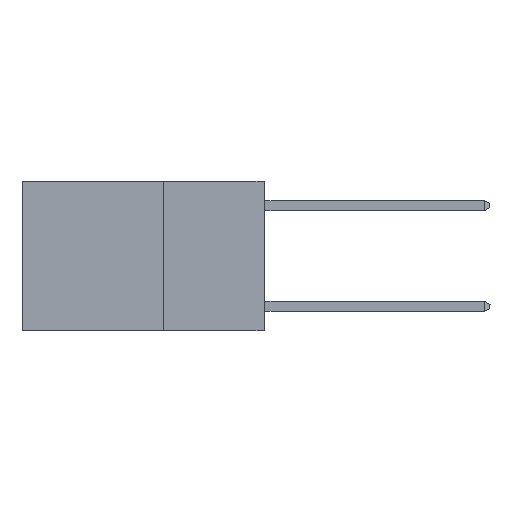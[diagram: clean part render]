
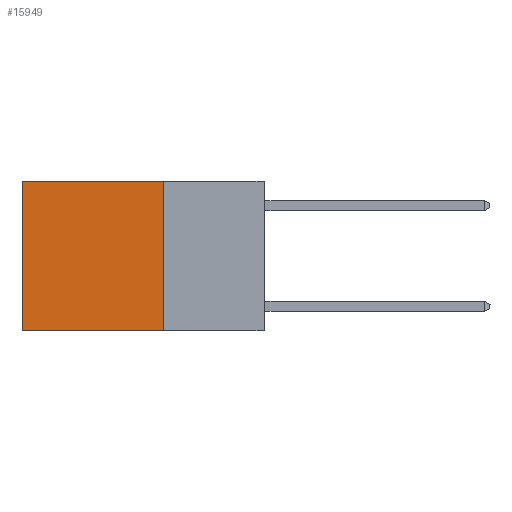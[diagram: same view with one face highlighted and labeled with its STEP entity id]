
A CAD part, left-side view. The second image highlights one B-rep face of the part: STEP entity #15949.
In plain terms, the highlighted planar face has unit normal (-1, 0, 0).
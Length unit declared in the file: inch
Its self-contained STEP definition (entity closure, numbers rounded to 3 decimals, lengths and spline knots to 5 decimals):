
#346 = CARTESIAN_POINT ( 'NONE',  ( 0.2625, 0.6, 0. ) ) ;
#1718 = DIRECTION ( 'NONE',  ( 0., 1., 0. ) ) ;
#1729 = ORIENTED_EDGE ( 'NONE', *, *, #13263, .F. ) ;
#2487 = ORIENTED_EDGE ( 'NONE', *, *, #10827, .F. ) ;
#2896 = DIRECTION ( 'NONE',  ( 0., 1., 0. ) ) ;
#3370 = VERTEX_POINT ( 'NONE', #15706 ) ;
#3487 = DIRECTION ( 'NONE',  ( 1., 0., 0. ) ) ;
#3703 = DIRECTION ( 'NONE',  ( 0., 0., -1. ) ) ;
#3858 = ORIENTED_EDGE ( 'NONE', *, *, #13022, .T. ) ;
#6907 = LINE ( 'NONE', #346, #17585 ) ;
#7411 = AXIS2_PLACEMENT_3D ( 'NONE', #15998, #3487, #13268 ) ;
#9078 = VECTOR ( 'NONE', #2896, 39.37008 ) ;
#9420 = VERTEX_POINT ( 'NONE', #12115 ) ;
#9879 = LINE ( 'NONE', #15665, #13117 ) ;
#9910 = LINE ( 'NONE', #11302, #9078 ) ;
#10001 = VECTOR ( 'NONE', #3703, 39.37008 ) ;
#10705 = EDGE_LOOP ( 'NONE', ( #3858, #2487, #1729, #12220 ) ) ;
#10827 = EDGE_CURVE ( 'NONE', #12619, #3370, #9910, .T. ) ;
#11302 = CARTESIAN_POINT ( 'NONE',  ( 0.2625, 0.25, -0.37 ) ) ;
#11639 = VERTEX_POINT ( 'NONE', #12858 ) ;
#11885 = PLANE ( 'NONE',  #7411 ) ;
#12115 = CARTESIAN_POINT ( 'NONE',  ( 0.2625, 0.6, 0. ) ) ;
#12220 = ORIENTED_EDGE ( 'NONE', *, *, #16415, .T. ) ;
#12619 = VERTEX_POINT ( 'NONE', #13543 ) ;
#12858 = CARTESIAN_POINT ( 'NONE',  ( 0.2625, 0.25, 0. ) ) ;
#12932 = DIRECTION ( 'NONE',  ( 0., 0., -1. ) ) ;
#13022 = EDGE_CURVE ( 'NONE', #9420, #3370, #6907, .T. ) ;
#13117 = VECTOR ( 'NONE', #1718, 39.37008 ) ;
#13263 = EDGE_CURVE ( 'NONE', #11639, #12619, #17794, .T. ) ;
#13268 = DIRECTION ( 'NONE',  ( 0., 0., -1. ) ) ;
#13462 = CARTESIAN_POINT ( 'NONE',  ( 0.2625, 0.25, 0. ) ) ;
#13543 = CARTESIAN_POINT ( 'NONE',  ( 0.2625, 0.25, -0.37 ) ) ;
#15665 = CARTESIAN_POINT ( 'NONE',  ( 0.2625, 0.25, 0. ) ) ;
#15706 = CARTESIAN_POINT ( 'NONE',  ( 0.2625, 0.6, -0.37 ) ) ;
#15949 = ADVANCED_FACE ( 'NONE', ( #17264 ), #11885, .F. ) ;
#15998 = CARTESIAN_POINT ( 'NONE',  ( 0.2625, 0.25, 0. ) ) ;
#16415 = EDGE_CURVE ( 'NONE', #11639, #9420, #9879, .T. ) ;
#17264 = FACE_OUTER_BOUND ( 'NONE', #10705, .T. ) ;
#17585 = VECTOR ( 'NONE', #12932, 39.37008 ) ;
#17794 = LINE ( 'NONE', #13462, #10001 ) ;
